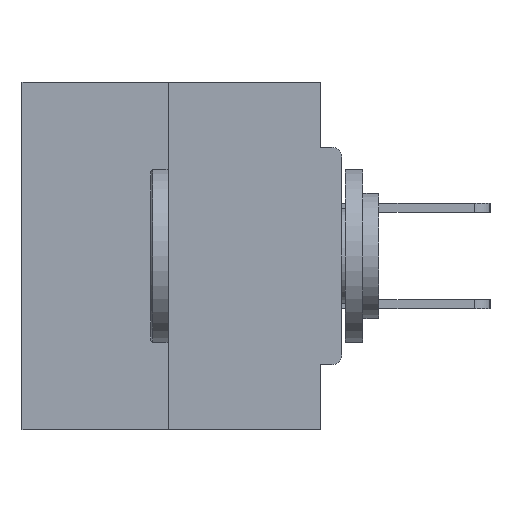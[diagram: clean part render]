
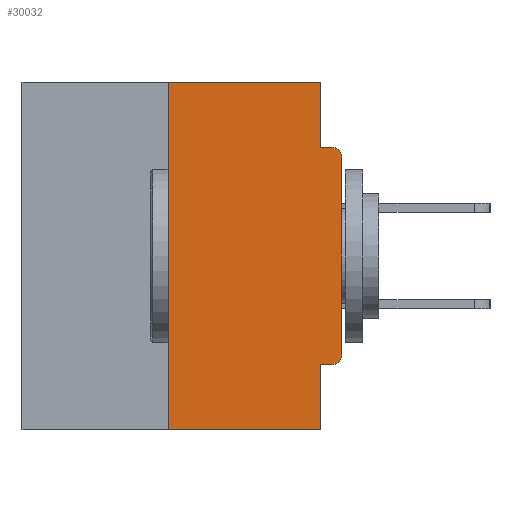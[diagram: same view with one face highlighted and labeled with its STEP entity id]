
A CAD part, left-side view. The second image highlights one B-rep face of the part: STEP entity #30032.
In plain terms, the highlighted planar face has unit normal (-1, 0, 0).
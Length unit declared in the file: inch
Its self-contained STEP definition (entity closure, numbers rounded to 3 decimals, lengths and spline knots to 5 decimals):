
#333 = LINE ( 'NONE', #5094, #25253 ) ;
#664 = VECTOR ( 'NONE', #35865, 39.37008 ) ;
#846 = CARTESIAN_POINT ( 'NONE',  ( 0., 0.031, 0. ) ) ;
#1323 = CARTESIAN_POINT ( 'NONE',  ( 0., 0.031, -0.4065 ) ) ;
#1692 = EDGE_CURVE ( 'NONE', #16821, #7964, #8690, .T. ) ;
#1862 = EDGE_LOOP ( 'NONE', ( #14132, #32769, #33251, #5404, #16457, #18572, #32627, #26322, #24181, #13907 ) ) ;
#1869 = EDGE_CURVE ( 'NONE', #31404, #32824, #23311, .T. ) ;
#2582 = CARTESIAN_POINT ( 'NONE',  ( 0., 0., 0. ) ) ;
#4204 = CARTESIAN_POINT ( 'NONE',  ( 0., 0.015, -0.3915 ) ) ;
#4435 = VECTOR ( 'NONE', #11168, 39.37008 ) ;
#4937 = EDGE_CURVE ( 'NONE', #17259, #27961, #19098, .T. ) ;
#5094 = CARTESIAN_POINT ( 'NONE',  ( 0., 0., -0.4065 ) ) ;
#5404 = ORIENTED_EDGE ( 'NONE', *, *, #13468, .F. ) ;
#5629 = CARTESIAN_POINT ( 'NONE',  ( 0., 0.25, 0. ) ) ;
#5649 = VECTOR ( 'NONE', #7610, 39.37008 ) ;
#5818 = CARTESIAN_POINT ( 'NONE',  ( 0., 0.46, 0. ) ) ;
#6278 = VECTOR ( 'NONE', #14074, 39.37008 ) ;
#6990 = DIRECTION ( 'NONE',  ( 0., 0., -1. ) ) ;
#7610 = DIRECTION ( 'NONE',  ( 0., -1., 0. ) ) ;
#7786 = CARTESIAN_POINT ( 'NONE',  ( 0., 0.25, 0. ) ) ;
#7964 = VERTEX_POINT ( 'NONE', #5629 ) ;
#8017 = DIRECTION ( 'NONE',  ( 0., 0., -1. ) ) ;
#8577 = DIRECTION ( 'NONE',  ( 1., 0., 0. ) ) ;
#8690 = LINE ( 'NONE', #7786, #664 ) ;
#9093 = EDGE_CURVE ( 'NONE', #10910, #22539, #333, .T. ) ;
#10910 = VERTEX_POINT ( 'NONE', #20280 ) ;
#11168 = DIRECTION ( 'NONE',  ( 0., 0., -1. ) ) ;
#11806 = CARTESIAN_POINT ( 'NONE',  ( 0., 0.031, -0.0935 ) ) ;
#12685 = CARTESIAN_POINT ( 'NONE',  ( 0., 0.015, -0.1085 ) ) ;
#12832 = CIRCLE ( 'NONE', #23107, 0.015 ) ;
#13468 = EDGE_CURVE ( 'NONE', #22539, #29313, #24523, .T. ) ;
#13812 = EDGE_CURVE ( 'NONE', #16821, #29313, #24316, .T. ) ;
#13907 = ORIENTED_EDGE ( 'NONE', *, *, #29993, .F. ) ;
#14074 = DIRECTION ( 'NONE',  ( 0., -1., 0. ) ) ;
#14132 = ORIENTED_EDGE ( 'NONE', *, *, #24909, .F. ) ;
#14230 = CARTESIAN_POINT ( 'NONE',  ( 0., 0.031, 0. ) ) ;
#14648 = VECTOR ( 'NONE', #16818, 39.37008 ) ;
#16063 = AXIS2_PLACEMENT_3D ( 'NONE', #12685, #20751, #6990 ) ;
#16457 = ORIENTED_EDGE ( 'NONE', *, *, #9093, .F. ) ;
#16818 = DIRECTION ( 'NONE',  ( 0., -1., 0. ) ) ;
#16821 = VERTEX_POINT ( 'NONE', #33407 ) ;
#17259 = VERTEX_POINT ( 'NONE', #11806 ) ;
#17592 = CARTESIAN_POINT ( 'NONE',  ( 0., 0., -0.1085 ) ) ;
#17707 = CIRCLE ( 'NONE', #16063, 0.015 ) ;
#17875 = AXIS2_PLACEMENT_3D ( 'NONE', #5818, #8577, #25311 ) ;
#18354 = DIRECTION ( 'NONE',  ( -1., 0., 0. ) ) ;
#18572 = ORIENTED_EDGE ( 'NONE', *, *, #21048, .T. ) ;
#19098 = LINE ( 'NONE', #34106, #14648 ) ;
#19175 = CARTESIAN_POINT ( 'NONE',  ( 0., 0.031, -0.5 ) ) ;
#19671 = CARTESIAN_POINT ( 'NONE',  ( 0., 0.46, 0. ) ) ;
#20280 = CARTESIAN_POINT ( 'NONE',  ( 0., 0.015, -0.4065 ) ) ;
#20751 = DIRECTION ( 'NONE',  ( -1., 0., 0. ) ) ;
#21048 = EDGE_CURVE ( 'NONE', #10910, #31404, #12832, .T. ) ;
#21400 = LINE ( 'NONE', #19671, #6278 ) ;
#22529 = DIRECTION ( 'NONE',  ( 0., 0., 1. ) ) ;
#22539 = VERTEX_POINT ( 'NONE', #1323 ) ;
#22790 = PLANE ( 'NONE',  #17875 ) ;
#23107 = AXIS2_PLACEMENT_3D ( 'NONE', #4204, #18354, #35247 ) ;
#23311 = LINE ( 'NONE', #2582, #31292 ) ;
#23630 = VECTOR ( 'NONE', #8017, 39.37008 ) ;
#24181 = ORIENTED_EDGE ( 'NONE', *, *, #4937, .F. ) ;
#24316 = LINE ( 'NONE', #24740, #5649 ) ;
#24523 = LINE ( 'NONE', #19175, #23630 ) ;
#24740 = CARTESIAN_POINT ( 'NONE',  ( 0., 0.46, -0.5 ) ) ;
#24909 = EDGE_CURVE ( 'NONE', #7964, #33020, #21400, .T. ) ;
#25253 = VECTOR ( 'NONE', #36041, 39.37008 ) ;
#25311 = DIRECTION ( 'NONE',  ( 0., 0., -1. ) ) ;
#25928 = EDGE_CURVE ( 'NONE', #32824, #27961, #17707, .T. ) ;
#26322 = ORIENTED_EDGE ( 'NONE', *, *, #25928, .T. ) ;
#27026 = FACE_OUTER_BOUND ( 'NONE', #1862, .T. ) ;
#27097 = CARTESIAN_POINT ( 'NONE',  ( 0., 0.015, -0.0935 ) ) ;
#27508 = CARTESIAN_POINT ( 'NONE',  ( 0., 0., -0.3915 ) ) ;
#27961 = VERTEX_POINT ( 'NONE', #27097 ) ;
#29313 = VERTEX_POINT ( 'NONE', #32675 ) ;
#29993 = EDGE_CURVE ( 'NONE', #33020, #17259, #35911, .T. ) ;
#30032 = ADVANCED_FACE ( 'NONE', ( #27026 ), #22790, .F. ) ;
#31292 = VECTOR ( 'NONE', #22529, 39.37008 ) ;
#31404 = VERTEX_POINT ( 'NONE', #27508 ) ;
#32627 = ORIENTED_EDGE ( 'NONE', *, *, #1869, .T. ) ;
#32675 = CARTESIAN_POINT ( 'NONE',  ( 0., 0.031, -0.5 ) ) ;
#32769 = ORIENTED_EDGE ( 'NONE', *, *, #1692, .F. ) ;
#32824 = VERTEX_POINT ( 'NONE', #17592 ) ;
#33020 = VERTEX_POINT ( 'NONE', #846 ) ;
#33251 = ORIENTED_EDGE ( 'NONE', *, *, #13812, .T. ) ;
#33407 = CARTESIAN_POINT ( 'NONE',  ( 0., 0.25, -0.5 ) ) ;
#34106 = CARTESIAN_POINT ( 'NONE',  ( 0., 0., -0.0935 ) ) ;
#35247 = DIRECTION ( 'NONE',  ( 0., 0., -1. ) ) ;
#35865 = DIRECTION ( 'NONE',  ( 0., 0., 1. ) ) ;
#35911 = LINE ( 'NONE', #14230, #4435 ) ;
#36041 = DIRECTION ( 'NONE',  ( 0., 1., 0. ) ) ;
